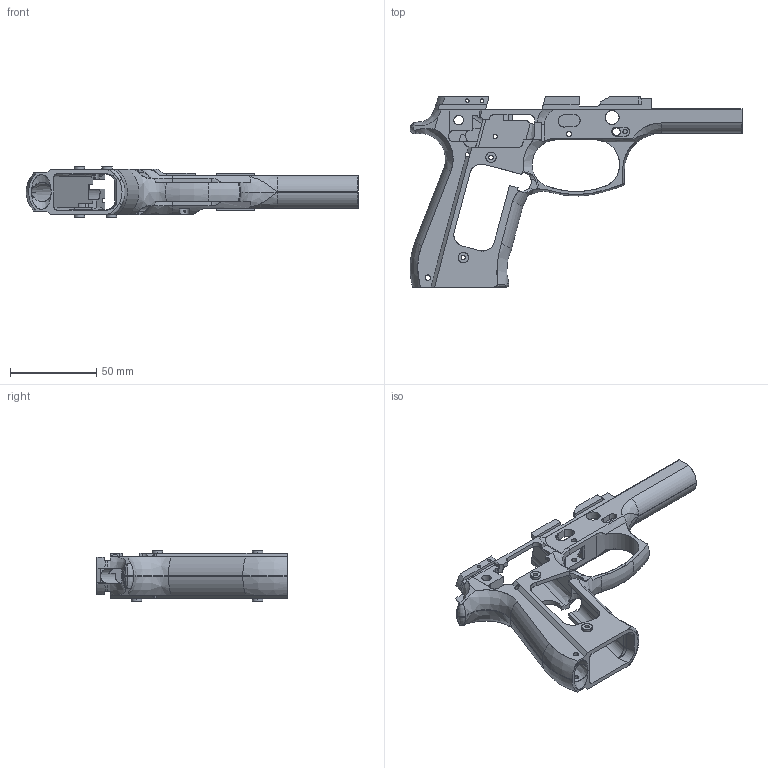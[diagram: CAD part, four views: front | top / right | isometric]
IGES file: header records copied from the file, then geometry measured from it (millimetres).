
Start section: SolidWorks IGES file using analytic representation for surfaces
Global section: file name: Beretta92FS.IGS; native system: SolidWorks 2005 by SolidWorks Corporation; preprocessor: SolidWorks 2005 by SolidWorks Corporation; author: Justin; date: 050326.231225; units: inch
Bounding box: 191.99 x 110.08 x 29.13 mm (x, y, z)
Surface area: 42925 mm2 (no closed solid volume)
Topology: 0 solids, 0 shells, 409 faces, 6263 edges, 6261 vertices
Faces by surface type: bspline 252, revolution 157
